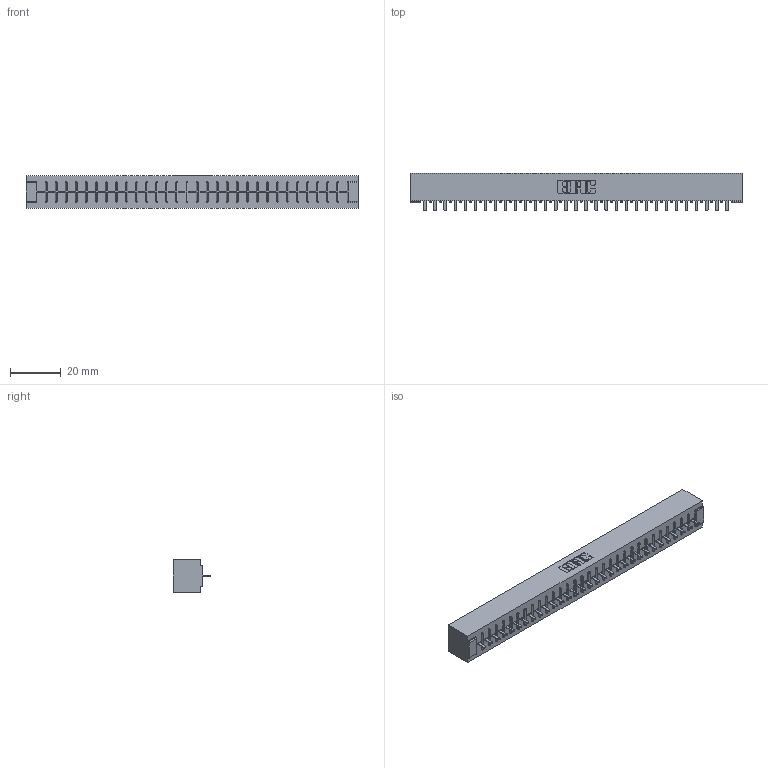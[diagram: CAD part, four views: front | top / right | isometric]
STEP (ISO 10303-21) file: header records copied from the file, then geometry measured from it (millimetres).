
FILE_DESCRIPTION (( 'STEP AP203' ), '1' );
FILE_NAME ('316-031-521-101.STEP', '2018-07-31T03:32:08', ( '' ), ( '' ), 'SwSTEP 2.0', 'SolidWorks 2016', '' );
FILE_SCHEMA (( 'CONFIG_CONTROL_DESIGN' ));
Length unit declared in the file: inch
Products named in the file (3): 306 Part_No Mounting; 306-290-001_121; 316-031-521-101
Assembly tree (32 placements, depth 2):
  316-031-521-101
    306 Part_No Mounting
    306-290-001_121  x31
Bounding box: 130.71 x 14.88 x 12.7 mm (x, y, z)
Volume: 14899.6 mm3; surface area: 15078.4 mm2
Topology: 32 solids, 32 shells, 2278 faces, 6399 edges, 4098 vertices
Faces by surface type: plane 1521, cylinder 633, sphere 124
Entity records: 30012 total; most frequent: CARTESIAN_POINT 5036, ORIENTED_EDGE 4990, DIRECTION 4967, EDGE_CURVE 2495, VECTOR 1949, LINE 1949, VERTEX_POINT 1578, AXIS2_PLACEMENT_3D 1509
